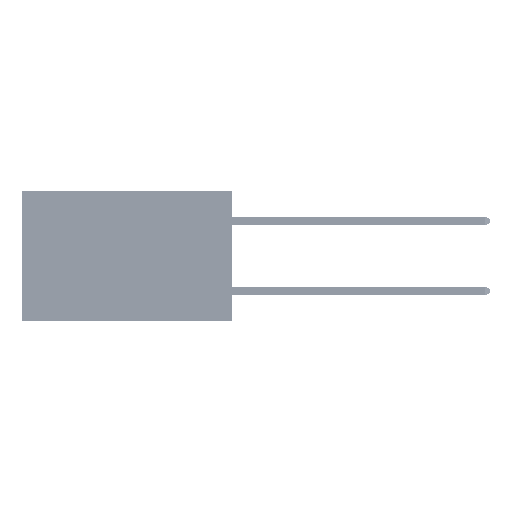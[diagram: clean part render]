
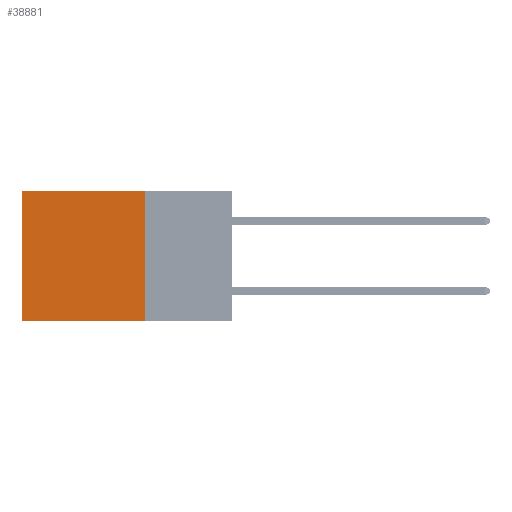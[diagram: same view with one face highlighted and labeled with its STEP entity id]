
A CAD part, left-side view. The second image highlights one B-rep face of the part: STEP entity #38881.
In plain terms, the highlighted planar face has unit normal (-1, 0, 0).
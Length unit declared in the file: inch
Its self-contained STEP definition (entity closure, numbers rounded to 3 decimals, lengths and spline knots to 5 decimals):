
#2210 = VECTOR ( 'NONE', #6917, 39.37008 ) ;
#6587 = DIRECTION ( 'NONE',  ( 0., 1., 0. ) ) ;
#6917 = DIRECTION ( 'NONE',  ( 0., 0., -1. ) ) ;
#7612 = CARTESIAN_POINT ( 'NONE',  ( 0.2875, 0.6, -0.37 ) ) ;
#9290 = PLANE ( 'NONE',  #23850 ) ;
#10218 = DIRECTION ( 'NONE',  ( 0., 1., 0. ) ) ;
#10532 = ORIENTED_EDGE ( 'NONE', *, *, #19567, .T. ) ;
#10707 = CARTESIAN_POINT ( 'NONE',  ( 0.2875, 0.25, 0. ) ) ;
#11778 = LINE ( 'NONE', #25870, #2210 ) ;
#13287 = DIRECTION ( 'NONE',  ( 1., 0., 0. ) ) ;
#13938 = DIRECTION ( 'NONE',  ( 0., 0., -1. ) ) ;
#14378 = EDGE_CURVE ( 'NONE', #45948, #14489, #47793, .T. ) ;
#14468 = LINE ( 'NONE', #10707, #22213 ) ;
#14489 = VERTEX_POINT ( 'NONE', #7612 ) ;
#16263 = VECTOR ( 'NONE', #13938, 39.37008 ) ;
#16586 = LINE ( 'NONE', #24858, #24306 ) ;
#19567 = EDGE_CURVE ( 'NONE', #26809, #45948, #14468, .T. ) ;
#21530 = CARTESIAN_POINT ( 'NONE',  ( 0.2875, 0.6, 0. ) ) ;
#22213 = VECTOR ( 'NONE', #6587, 39.37008 ) ;
#23850 = AXIS2_PLACEMENT_3D ( 'NONE', #35902, #13287, #36395 ) ;
#24306 = VECTOR ( 'NONE', #10218, 39.37008 ) ;
#24626 = EDGE_CURVE ( 'NONE', #26809, #49190, #11778, .T. ) ;
#24858 = CARTESIAN_POINT ( 'NONE',  ( 0.2875, 0.25, -0.37 ) ) ;
#25870 = CARTESIAN_POINT ( 'NONE',  ( 0.2875, 0.25, 0. ) ) ;
#26809 = VERTEX_POINT ( 'NONE', #42352 ) ;
#33005 = ORIENTED_EDGE ( 'NONE', *, *, #40892, .F. ) ;
#33584 = ORIENTED_EDGE ( 'NONE', *, *, #14378, .T. ) ;
#35902 = CARTESIAN_POINT ( 'NONE',  ( 0.2875, 0.25, 0. ) ) ;
#36395 = DIRECTION ( 'NONE',  ( 0., 0., -1. ) ) ;
#38881 = ADVANCED_FACE ( 'NONE', ( #39404 ), #9290, .F. ) ;
#39404 = FACE_OUTER_BOUND ( 'NONE', #42910, .T. ) ;
#40656 = ORIENTED_EDGE ( 'NONE', *, *, #24626, .F. ) ;
#40892 = EDGE_CURVE ( 'NONE', #49190, #14489, #16586, .T. ) ;
#42352 = CARTESIAN_POINT ( 'NONE',  ( 0.2875, 0.25, 0. ) ) ;
#42910 = EDGE_LOOP ( 'NONE', ( #33584, #33005, #40656, #10532 ) ) ;
#45948 = VERTEX_POINT ( 'NONE', #21530 ) ;
#47793 = LINE ( 'NONE', #48032, #16263 ) ;
#48032 = CARTESIAN_POINT ( 'NONE',  ( 0.2875, 0.6, 0. ) ) ;
#48285 = CARTESIAN_POINT ( 'NONE',  ( 0.2875, 0.25, -0.37 ) ) ;
#49190 = VERTEX_POINT ( 'NONE', #48285 ) ;
